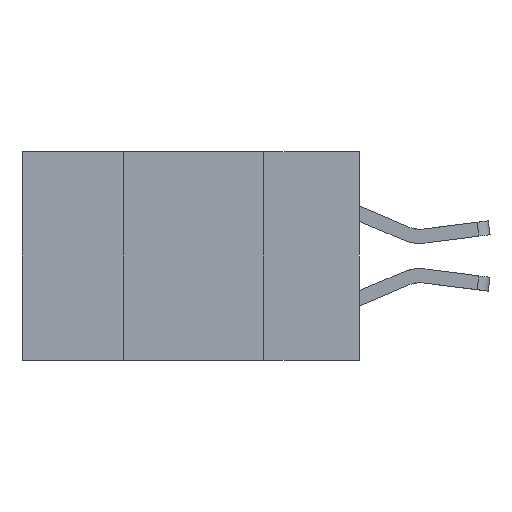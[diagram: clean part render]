
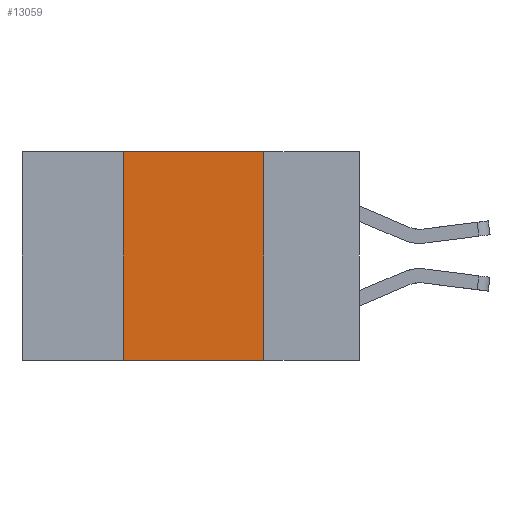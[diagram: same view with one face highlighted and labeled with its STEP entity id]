
A CAD part, left-side view. The second image highlights one B-rep face of the part: STEP entity #13059.
In plain terms, the highlighted planar face has unit normal (-1, 0, 0).
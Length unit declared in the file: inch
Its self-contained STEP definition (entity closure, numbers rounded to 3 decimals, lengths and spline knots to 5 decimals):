
#1177 = VERTEX_POINT ( 'NONE', #12797 ) ;
#1795 = DIRECTION ( 'NONE',  ( 0., 0., -1. ) ) ;
#1957 = CARTESIAN_POINT ( 'NONE',  ( 0., 0.17, -0.37 ) ) ;
#2253 = ORIENTED_EDGE ( 'NONE', *, *, #7483, .F. ) ;
#2274 = DIRECTION ( 'NONE',  ( 0., 0., -1. ) ) ;
#2929 = CARTESIAN_POINT ( 'NONE',  ( 0., 0.6, 0. ) ) ;
#3382 = CARTESIAN_POINT ( 'NONE',  ( 0., 0.42, 0. ) ) ;
#3383 = VERTEX_POINT ( 'NONE', #7379 ) ;
#3894 = ORIENTED_EDGE ( 'NONE', *, *, #6377, .F. ) ;
#4090 = EDGE_CURVE ( 'NONE', #6252, #8981, #5684, .T. ) ;
#5626 = EDGE_CURVE ( 'NONE', #6252, #3383, #7676, .T. ) ;
#5684 = LINE ( 'NONE', #13209, #14559 ) ;
#6211 = DIRECTION ( 'NONE',  ( 0., -1., 0. ) ) ;
#6252 = VERTEX_POINT ( 'NONE', #6679 ) ;
#6377 = EDGE_CURVE ( 'NONE', #1177, #8981, #9698, .T. ) ;
#6679 = CARTESIAN_POINT ( 'NONE',  ( 0., 0.42, -0.37 ) ) ;
#7317 = DIRECTION ( 'NONE',  ( 0., -1., 0. ) ) ;
#7379 = CARTESIAN_POINT ( 'NONE',  ( 0., 0.42, 0. ) ) ;
#7483 = EDGE_CURVE ( 'NONE', #3383, #1177, #8770, .T. ) ;
#7592 = PLANE ( 'NONE',  #11650 ) ;
#7676 = LINE ( 'NONE', #3382, #11140 ) ;
#8103 = CARTESIAN_POINT ( 'NONE',  ( 0., 0.17, 0. ) ) ;
#8395 = VECTOR ( 'NONE', #7317, 39.37008 ) ;
#8543 = CARTESIAN_POINT ( 'NONE',  ( 0., 0.6, 0. ) ) ;
#8770 = LINE ( 'NONE', #8543, #8395 ) ;
#8805 = DIRECTION ( 'NONE',  ( 1., 0., 0. ) ) ;
#8981 = VERTEX_POINT ( 'NONE', #1957 ) ;
#9006 = ORIENTED_EDGE ( 'NONE', *, *, #5626, .F. ) ;
#9698 = LINE ( 'NONE', #8103, #12404 ) ;
#9734 = ORIENTED_EDGE ( 'NONE', *, *, #4090, .T. ) ;
#11140 = VECTOR ( 'NONE', #11511, 39.37008 ) ;
#11484 = EDGE_LOOP ( 'NONE', ( #3894, #2253, #9006, #9734 ) ) ;
#11511 = DIRECTION ( 'NONE',  ( 0., 0., 1. ) ) ;
#11650 = AXIS2_PLACEMENT_3D ( 'NONE', #2929, #8805, #1795 ) ;
#12404 = VECTOR ( 'NONE', #2274, 39.37008 ) ;
#12797 = CARTESIAN_POINT ( 'NONE',  ( 0., 0.17, 0. ) ) ;
#13059 = ADVANCED_FACE ( 'NONE', ( #13663 ), #7592, .F. ) ;
#13209 = CARTESIAN_POINT ( 'NONE',  ( 0., 0.6, -0.37 ) ) ;
#13663 = FACE_OUTER_BOUND ( 'NONE', #11484, .T. ) ;
#14559 = VECTOR ( 'NONE', #6211, 39.37008 ) ;
